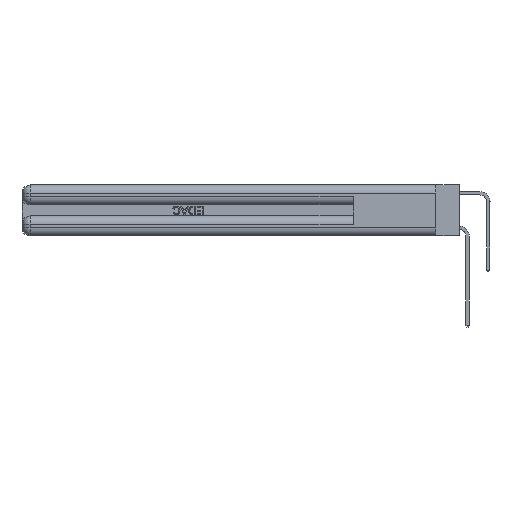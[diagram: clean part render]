
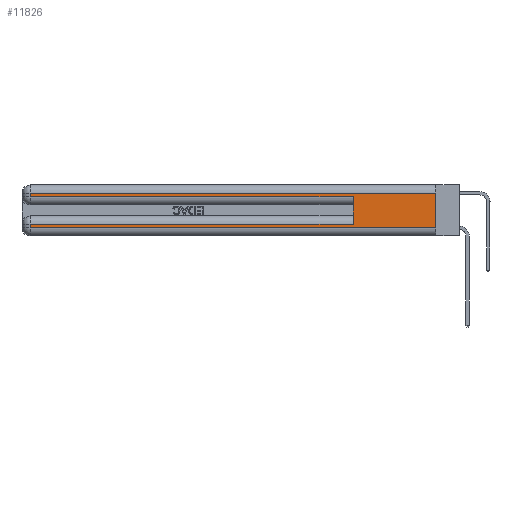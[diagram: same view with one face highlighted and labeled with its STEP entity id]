
A CAD part, left-side view. The second image highlights one B-rep face of the part: STEP entity #11826.
In plain terms, the highlighted planar face has unit normal (-1, 0, 0).
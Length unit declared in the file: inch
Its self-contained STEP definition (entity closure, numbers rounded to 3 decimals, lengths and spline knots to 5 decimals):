
#864 = VECTOR ( 'NONE', #15381, 39.37008 ) ;
#1127 = EDGE_CURVE ( 'NONE', #2384, #12107, #15298, .T. ) ;
#1315 = CARTESIAN_POINT ( 'NONE',  ( 0., 2.94, 0.06 ) ) ;
#1946 = ORIENTED_EDGE ( 'NONE', *, *, #30842, .T. ) ;
#2348 = ORIENTED_EDGE ( 'NONE', *, *, #1127, .T. ) ;
#2384 = VERTEX_POINT ( 'NONE', #16805 ) ;
#3258 = EDGE_CURVE ( 'NONE', #12724, #11919, #21687, .T. ) ;
#3733 = DIRECTION ( 'NONE',  ( 0., 0., -1. ) ) ;
#4303 = CARTESIAN_POINT ( 'NONE',  ( 0., 2.94, 0.085 ) ) ;
#4583 = VECTOR ( 'NONE', #16916, 39.37008 ) ;
#5201 = LINE ( 'NONE', #31979, #33532 ) ;
#5635 = CARTESIAN_POINT ( 'NONE',  ( 0., 0.6, 0.085 ) ) ;
#5989 = CARTESIAN_POINT ( 'NONE',  ( 0., 0., 0.31 ) ) ;
#6231 = VERTEX_POINT ( 'NONE', #32376 ) ;
#6959 = ORIENTED_EDGE ( 'NONE', *, *, #14836, .F. ) ;
#8355 = ORIENTED_EDGE ( 'NONE', *, *, #12833, .T. ) ;
#8817 = DIRECTION ( 'NONE',  ( 0., 1., 0. ) ) ;
#9019 = DIRECTION ( 'NONE',  ( 1., 0., 0. ) ) ;
#9129 = VECTOR ( 'NONE', #14875, 39.37008 ) ;
#10104 = DIRECTION ( 'NONE',  ( 0., 0., -1. ) ) ;
#11316 = LINE ( 'NONE', #5989, #14693 ) ;
#11597 = LINE ( 'NONE', #28607, #32726 ) ;
#11745 = VERTEX_POINT ( 'NONE', #14759 ) ;
#11826 = ADVANCED_FACE ( 'NONE', ( #25779 ), #33402, .F. ) ;
#11919 = VERTEX_POINT ( 'NONE', #1315 ) ;
#12043 = ORIENTED_EDGE ( 'NONE', *, *, #19013, .F. ) ;
#12107 = VERTEX_POINT ( 'NONE', #32408 ) ;
#12724 = VERTEX_POINT ( 'NONE', #4303 ) ;
#12833 = EDGE_CURVE ( 'NONE', #11919, #13915, #31618, .T. ) ;
#13438 = ORIENTED_EDGE ( 'NONE', *, *, #3258, .T. ) ;
#13813 = CARTESIAN_POINT ( 'NONE',  ( 0., 0., 0.06 ) ) ;
#13915 = VERTEX_POINT ( 'NONE', #14233 ) ;
#14233 = CARTESIAN_POINT ( 'NONE',  ( 0., 0., 0.06 ) ) ;
#14636 = CARTESIAN_POINT ( 'NONE',  ( 0., 2.94, 0.37 ) ) ;
#14693 = VECTOR ( 'NONE', #8817, 39.37008 ) ;
#14759 = CARTESIAN_POINT ( 'NONE',  ( 0., 0., 0.31 ) ) ;
#14836 = EDGE_CURVE ( 'NONE', #15505, #12107, #15312, .T. ) ;
#14875 = DIRECTION ( 'NONE',  ( 0., 0., -1. ) ) ;
#15202 = CARTESIAN_POINT ( 'NONE',  ( 0., 2.94, 0.37 ) ) ;
#15298 = LINE ( 'NONE', #25877, #864 ) ;
#15312 = LINE ( 'NONE', #34548, #20361 ) ;
#15381 = DIRECTION ( 'NONE',  ( 0., -1., 0. ) ) ;
#15505 = VERTEX_POINT ( 'NONE', #5635 ) ;
#16667 = EDGE_CURVE ( 'NONE', #6231, #2384, #28576, .T. ) ;
#16752 = ORIENTED_EDGE ( 'NONE', *, *, #22821, .T. ) ;
#16805 = CARTESIAN_POINT ( 'NONE',  ( 0., 2.94, 0.285 ) ) ;
#16916 = DIRECTION ( 'NONE',  ( 0., -1., 0. ) ) ;
#19013 = EDGE_CURVE ( 'NONE', #11745, #13915, #5201, .T. ) ;
#20361 = VECTOR ( 'NONE', #20919, 39.37008 ) ;
#20919 = DIRECTION ( 'NONE',  ( 0., 0., 1. ) ) ;
#21687 = LINE ( 'NONE', #15202, #31385 ) ;
#22821 = EDGE_CURVE ( 'NONE', #11745, #6231, #11316, .T. ) ;
#25185 = CARTESIAN_POINT ( 'NONE',  ( 0., 0., 0.37 ) ) ;
#25230 = EDGE_LOOP ( 'NONE', ( #12043, #16752, #29982, #2348, #6959, #1946, #13438, #8355 ) ) ;
#25779 = FACE_OUTER_BOUND ( 'NONE', #25230, .T. ) ;
#25877 = CARTESIAN_POINT ( 'NONE',  ( 0., 0., 0.285 ) ) ;
#26645 = AXIS2_PLACEMENT_3D ( 'NONE', #25185, #9019, #3733 ) ;
#28576 = LINE ( 'NONE', #14636, #9129 ) ;
#28607 = CARTESIAN_POINT ( 'NONE',  ( 0., 0., 0.085 ) ) ;
#29119 = DIRECTION ( 'NONE',  ( 0., 0., -1. ) ) ;
#29982 = ORIENTED_EDGE ( 'NONE', *, *, #16667, .T. ) ;
#30842 = EDGE_CURVE ( 'NONE', #15505, #12724, #11597, .T. ) ;
#31385 = VECTOR ( 'NONE', #29119, 39.37008 ) ;
#31618 = LINE ( 'NONE', #13813, #4583 ) ;
#31979 = CARTESIAN_POINT ( 'NONE',  ( 0., 0., 0.37 ) ) ;
#32376 = CARTESIAN_POINT ( 'NONE',  ( 0., 2.94, 0.31 ) ) ;
#32408 = CARTESIAN_POINT ( 'NONE',  ( 0., 0.6, 0.285 ) ) ;
#32726 = VECTOR ( 'NONE', #33965, 39.37008 ) ;
#33402 = PLANE ( 'NONE',  #26645 ) ;
#33532 = VECTOR ( 'NONE', #10104, 39.37008 ) ;
#33965 = DIRECTION ( 'NONE',  ( 0., 1., 0. ) ) ;
#34548 = CARTESIAN_POINT ( 'NONE',  ( 0., 0.6, 0.145 ) ) ;
